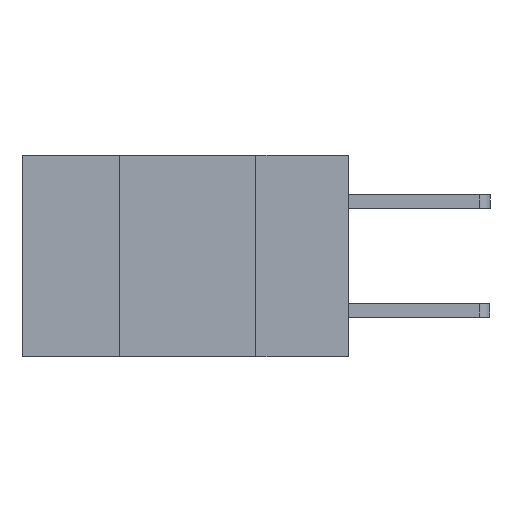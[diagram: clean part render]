
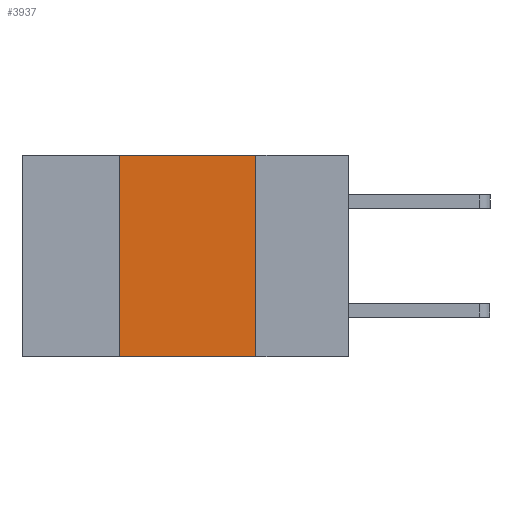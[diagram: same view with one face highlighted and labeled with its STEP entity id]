
A CAD part, left-side view. The second image highlights one B-rep face of the part: STEP entity #3937.
In plain terms, the highlighted planar face has unit normal (-1, 0, 0).
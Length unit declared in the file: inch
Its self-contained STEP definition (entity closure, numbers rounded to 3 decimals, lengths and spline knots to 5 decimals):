
#567 = LINE ( 'NONE', #5676, #5161 ) ;
#637 = VECTOR ( 'NONE', #10000, 39.37008 ) ;
#905 = DIRECTION ( 'NONE',  ( 0., 0., -1. ) ) ;
#962 = EDGE_LOOP ( 'NONE', ( #9608, #6097, #5517, #3840 ) ) ;
#1064 = DIRECTION ( 'NONE',  ( 0., -1., 0. ) ) ;
#1323 = EDGE_CURVE ( 'NONE', #8281, #2495, #567, .T. ) ;
#1359 = FACE_OUTER_BOUND ( 'NONE', #962, .T. ) ;
#2361 = VECTOR ( 'NONE', #1064, 39.37008 ) ;
#2495 = VERTEX_POINT ( 'NONE', #10077 ) ;
#3636 = CARTESIAN_POINT ( 'NONE',  ( 0., 0.6, -0.37 ) ) ;
#3840 = ORIENTED_EDGE ( 'NONE', *, *, #7407, .T. ) ;
#3937 = ADVANCED_FACE ( 'NONE', ( #1359 ), #6759, .F. ) ;
#4822 = CARTESIAN_POINT ( 'NONE',  ( 0., 0.42, -0.37 ) ) ;
#4941 = LINE ( 'NONE', #3636, #637 ) ;
#5161 = VECTOR ( 'NONE', #905, 39.37008 ) ;
#5517 = ORIENTED_EDGE ( 'NONE', *, *, #10418, .F. ) ;
#5646 = CARTESIAN_POINT ( 'NONE',  ( 0., 0.6, 0. ) ) ;
#5676 = CARTESIAN_POINT ( 'NONE',  ( 0., 0.17, 0. ) ) ;
#6097 = ORIENTED_EDGE ( 'NONE', *, *, #8837, .F. ) ;
#6429 = LINE ( 'NONE', #9650, #11000 ) ;
#6665 = DIRECTION ( 'NONE',  ( 0., 0., -1. ) ) ;
#6674 = DIRECTION ( 'NONE',  ( 1., 0., 0. ) ) ;
#6759 = PLANE ( 'NONE',  #7034 ) ;
#6899 = CARTESIAN_POINT ( 'NONE',  ( 0., 0.6, 0. ) ) ;
#7034 = AXIS2_PLACEMENT_3D ( 'NONE', #6899, #6674, #6665 ) ;
#7407 = EDGE_CURVE ( 'NONE', #7651, #2495, #4941, .T. ) ;
#7651 = VERTEX_POINT ( 'NONE', #4822 ) ;
#8172 = VERTEX_POINT ( 'NONE', #9334 ) ;
#8281 = VERTEX_POINT ( 'NONE', #11291 ) ;
#8837 = EDGE_CURVE ( 'NONE', #8172, #8281, #9660, .T. ) ;
#9334 = CARTESIAN_POINT ( 'NONE',  ( 0., 0.42, 0. ) ) ;
#9608 = ORIENTED_EDGE ( 'NONE', *, *, #1323, .F. ) ;
#9650 = CARTESIAN_POINT ( 'NONE',  ( 0., 0.42, 0. ) ) ;
#9660 = LINE ( 'NONE', #5646, #2361 ) ;
#10000 = DIRECTION ( 'NONE',  ( 0., -1., 0. ) ) ;
#10077 = CARTESIAN_POINT ( 'NONE',  ( 0., 0.17, -0.37 ) ) ;
#10418 = EDGE_CURVE ( 'NONE', #7651, #8172, #6429, .T. ) ;
#11000 = VECTOR ( 'NONE', #11447, 39.37008 ) ;
#11291 = CARTESIAN_POINT ( 'NONE',  ( 0., 0.17, 0. ) ) ;
#11447 = DIRECTION ( 'NONE',  ( 0., 0., 1. ) ) ;
